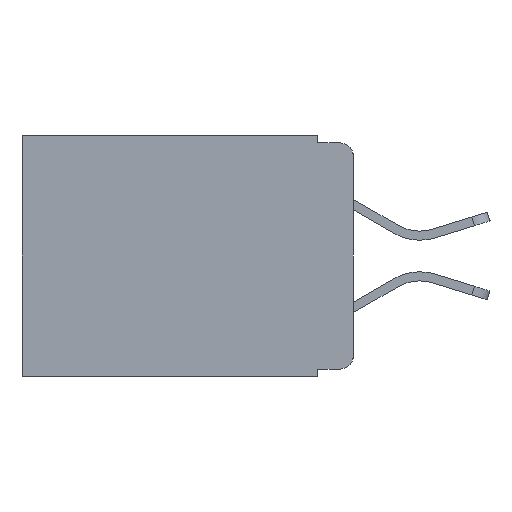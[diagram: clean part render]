
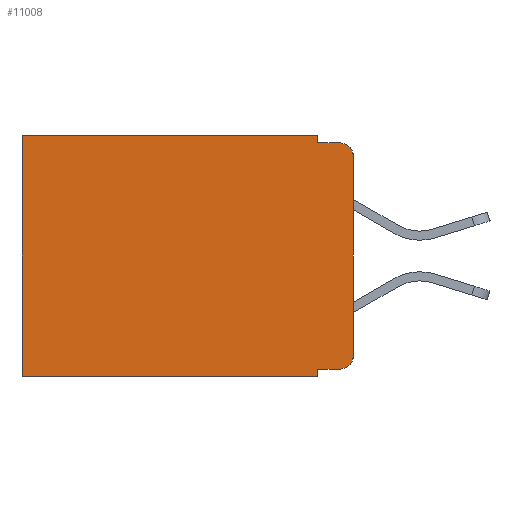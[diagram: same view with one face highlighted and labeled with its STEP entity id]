
A CAD part, left-side view. The second image highlights one B-rep face of the part: STEP entity #11008.
In plain terms, the highlighted planar face has unit normal (-1, 0, 0).
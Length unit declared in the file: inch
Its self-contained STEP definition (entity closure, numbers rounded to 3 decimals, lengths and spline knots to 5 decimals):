
#55 = ORIENTED_EDGE ( 'NONE', *, *, #11494, .F. ) ;
#74 = LINE ( 'NONE', #10347, #13926 ) ;
#613 = LINE ( 'NONE', #19935, #10305 ) ;
#948 = CARTESIAN_POINT ( 'NONE',  ( 0.298, 0., -0.03 ) ) ;
#1304 = CARTESIAN_POINT ( 'NONE',  ( 0.298, 0.02, -0.313 ) ) ;
#2139 = CIRCLE ( 'NONE', #2442, 0.02 ) ;
#2442 = AXIS2_PLACEMENT_3D ( 'NONE', #5671, #17883, #7450 ) ;
#2463 = CARTESIAN_POINT ( 'NONE',  ( 0.298, 0.051, 0. ) ) ;
#2634 = CARTESIAN_POINT ( 'NONE',  ( 0.298, 0.02, -0.333 ) ) ;
#2682 = VERTEX_POINT ( 'NONE', #21706 ) ;
#3218 = DIRECTION ( 'NONE',  ( 0., 0., -1. ) ) ;
#3316 = CARTESIAN_POINT ( 'NONE',  ( 0.298, 0., 0. ) ) ;
#3451 = EDGE_CURVE ( 'NONE', #16812, #2682, #22135, .T. ) ;
#3830 = VECTOR ( 'NONE', #10375, 39.37008 ) ;
#3871 = CARTESIAN_POINT ( 'NONE',  ( 0.298, 0.051, 0. ) ) ;
#3946 = VERTEX_POINT ( 'NONE', #948 ) ;
#4415 = LINE ( 'NONE', #19051, #3830 ) ;
#4547 = EDGE_LOOP ( 'NONE', ( #9181, #14922, #13138, #10425, #7360, #19540, #55, #12386, #15069, #4936 ) ) ;
#4775 = LINE ( 'NONE', #3871, #18195 ) ;
#4936 = ORIENTED_EDGE ( 'NONE', *, *, #22113, .T. ) ;
#5203 = DIRECTION ( 'NONE',  ( 0., 0., -1. ) ) ;
#5237 = VERTEX_POINT ( 'NONE', #10124 ) ;
#5671 = CARTESIAN_POINT ( 'NONE',  ( 0.298, 0.02, -0.03 ) ) ;
#6406 = VERTEX_POINT ( 'NONE', #7951 ) ;
#7023 = EDGE_CURVE ( 'NONE', #5237, #13979, #15836, .T. ) ;
#7139 = CARTESIAN_POINT ( 'NONE',  ( 0.298, 0.02, -0.01 ) ) ;
#7360 = ORIENTED_EDGE ( 'NONE', *, *, #3451, .T. ) ;
#7446 = EDGE_CURVE ( 'NONE', #3946, #9205, #2139, .T. ) ;
#7450 = DIRECTION ( 'NONE',  ( 0., 0., -1. ) ) ;
#7506 = DIRECTION ( 'NONE',  ( 0., 0., -1. ) ) ;
#7793 = DIRECTION ( 'NONE',  ( 0., -1., 0. ) ) ;
#7951 = CARTESIAN_POINT ( 'NONE',  ( 0.298, 0.473, -0.343 ) ) ;
#8178 = EDGE_CURVE ( 'NONE', #18767, #9205, #613, .T. ) ;
#8925 = EDGE_CURVE ( 'NONE', #5237, #10812, #21128, .T. ) ;
#9181 = ORIENTED_EDGE ( 'NONE', *, *, #9777, .F. ) ;
#9205 = VERTEX_POINT ( 'NONE', #7139 ) ;
#9250 = DIRECTION ( 'NONE',  ( 0., 1., 0. ) ) ;
#9354 = VECTOR ( 'NONE', #10014, 39.37008 ) ;
#9777 = EDGE_CURVE ( 'NONE', #3946, #10638, #4415, .T. ) ;
#9884 = DIRECTION ( 'NONE',  ( 0., -1., 0. ) ) ;
#10014 = DIRECTION ( 'NONE',  ( 0., 1., 0. ) ) ;
#10099 = CARTESIAN_POINT ( 'NONE',  ( 0.298, 0.051, -0.01 ) ) ;
#10124 = CARTESIAN_POINT ( 'NONE',  ( 0.298, 0.051, -0.333 ) ) ;
#10305 = VECTOR ( 'NONE', #7793, 39.37008 ) ;
#10347 = CARTESIAN_POINT ( 'NONE',  ( 0.298, 0.473, 0. ) ) ;
#10375 = DIRECTION ( 'NONE',  ( 0., 0., -1. ) ) ;
#10425 = ORIENTED_EDGE ( 'NONE', *, *, #20247, .F. ) ;
#10624 = VECTOR ( 'NONE', #21787, 39.37008 ) ;
#10638 = VERTEX_POINT ( 'NONE', #12869 ) ;
#10812 = VERTEX_POINT ( 'NONE', #2634 ) ;
#11008 = ADVANCED_FACE ( 'NONE', ( #19404 ), #13942, .F. ) ;
#11494 = EDGE_CURVE ( 'NONE', #13979, #6406, #18599, .T. ) ;
#12183 = DIRECTION ( 'NONE',  ( 0., 0., -1. ) ) ;
#12386 = ORIENTED_EDGE ( 'NONE', *, *, #7023, .F. ) ;
#12844 = EDGE_CURVE ( 'NONE', #2682, #6406, #74, .T. ) ;
#12869 = CARTESIAN_POINT ( 'NONE',  ( 0.298, 0., -0.313 ) ) ;
#13097 = CARTESIAN_POINT ( 'NONE',  ( 0.298, 0.051, 0. ) ) ;
#13138 = ORIENTED_EDGE ( 'NONE', *, *, #8178, .F. ) ;
#13859 = DIRECTION ( 'NONE',  ( -1., 0., 0. ) ) ;
#13926 = VECTOR ( 'NONE', #12183, 39.37008 ) ;
#13942 = PLANE ( 'NONE',  #22390 ) ;
#13979 = VERTEX_POINT ( 'NONE', #21358 ) ;
#14703 = AXIS2_PLACEMENT_3D ( 'NONE', #1304, #13859, #3218 ) ;
#14834 = CIRCLE ( 'NONE', #14703, 0.02 ) ;
#14922 = ORIENTED_EDGE ( 'NONE', *, *, #7446, .T. ) ;
#15069 = ORIENTED_EDGE ( 'NONE', *, *, #8925, .T. ) ;
#15692 = DIRECTION ( 'NONE',  ( 1., 0., 0. ) ) ;
#15836 = LINE ( 'NONE', #13097, #10624 ) ;
#16532 = VECTOR ( 'NONE', #9884, 39.37008 ) ;
#16812 = VERTEX_POINT ( 'NONE', #2463 ) ;
#17580 = VECTOR ( 'NONE', #9250, 39.37008 ) ;
#17883 = DIRECTION ( 'NONE',  ( -1., 0., 0. ) ) ;
#18195 = VECTOR ( 'NONE', #7506, 39.37008 ) ;
#18544 = CARTESIAN_POINT ( 'NONE',  ( 0.298, 0.051, -0.333 ) ) ;
#18599 = LINE ( 'NONE', #22206, #9354 ) ;
#18767 = VERTEX_POINT ( 'NONE', #10099 ) ;
#19051 = CARTESIAN_POINT ( 'NONE',  ( 0.298, 0., 0. ) ) ;
#19404 = FACE_OUTER_BOUND ( 'NONE', #4547, .T. ) ;
#19540 = ORIENTED_EDGE ( 'NONE', *, *, #12844, .T. ) ;
#19935 = CARTESIAN_POINT ( 'NONE',  ( 0.298, 0.051, -0.01 ) ) ;
#20247 = EDGE_CURVE ( 'NONE', #16812, #18767, #4775, .T. ) ;
#21128 = LINE ( 'NONE', #18544, #16532 ) ;
#21358 = CARTESIAN_POINT ( 'NONE',  ( 0.298, 0.051, -0.343 ) ) ;
#21706 = CARTESIAN_POINT ( 'NONE',  ( 0.298, 0.473, 0. ) ) ;
#21787 = DIRECTION ( 'NONE',  ( 0., 0., -1. ) ) ;
#22113 = EDGE_CURVE ( 'NONE', #10812, #10638, #14834, .T. ) ;
#22135 = LINE ( 'NONE', #22591, #17580 ) ;
#22206 = CARTESIAN_POINT ( 'NONE',  ( 0.298, 0., -0.343 ) ) ;
#22390 = AXIS2_PLACEMENT_3D ( 'NONE', #3316, #15692, #5203 ) ;
#22591 = CARTESIAN_POINT ( 'NONE',  ( 0.298, 0., 0. ) ) ;
